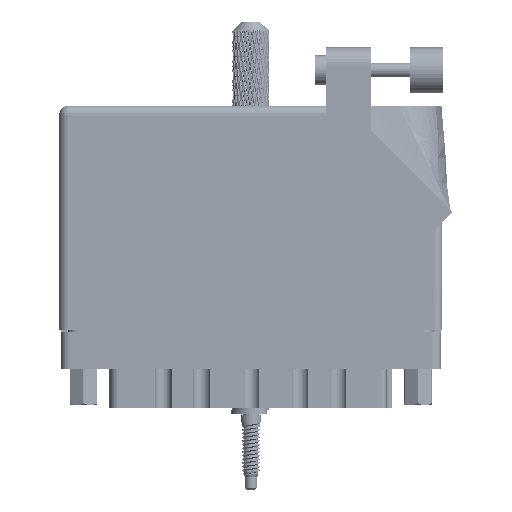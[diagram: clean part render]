
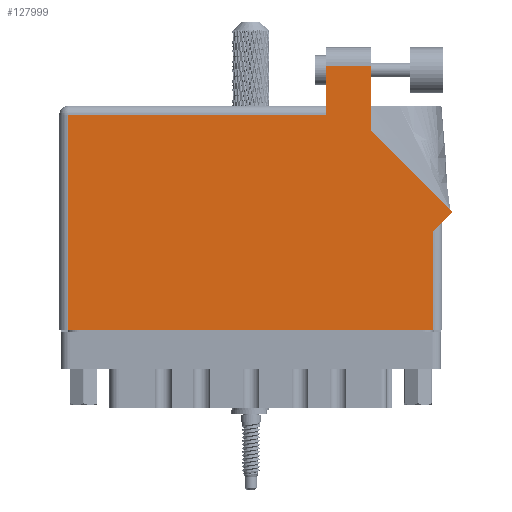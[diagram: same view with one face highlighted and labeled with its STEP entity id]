
A CAD part, front view. The second image highlights one B-rep face of the part: STEP entity #127999.
In plain terms, the highlighted face is planar.
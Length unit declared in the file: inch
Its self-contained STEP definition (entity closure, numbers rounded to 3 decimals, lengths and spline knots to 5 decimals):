
#1914 = DIRECTION ( 'NONE',  ( -1., 0., 0. ) ) ;
#2502 = VECTOR ( 'NONE', #121194, 39.37008 ) ;
#2871 = PLANE ( 'NONE',  #20234 ) ;
#4360 = VERTEX_POINT ( 'NONE', #15477 ) ;
#4693 = ORIENTED_EDGE ( 'NONE', *, *, #49996, .T. ) ;
#5023 = VERTEX_POINT ( 'NONE', #49099 ) ;
#8098 = LINE ( 'NONE', #32141, #100807 ) ;
#8764 = CARTESIAN_POINT ( 'NONE',  ( 1.819, 1.53, 0. ) ) ;
#9034 = VECTOR ( 'NONE', #18438, 39.37008 ) ;
#14349 = FACE_OUTER_BOUND ( 'NONE', #124347, .T. ) ;
#15477 = CARTESIAN_POINT ( 'NONE',  ( 1.819, 1.468, 0. ) ) ;
#15660 = VERTEX_POINT ( 'NONE', #127112 ) ;
#16513 = CARTESIAN_POINT ( 'NONE',  ( 0.062, 0., 0. ) ) ;
#18438 = DIRECTION ( 'NONE',  ( 1., 0., 0. ) ) ;
#19070 = VECTOR ( 'NONE', #127093, 39.37008 ) ;
#20234 = AXIS2_PLACEMENT_3D ( 'NONE', #71954, #51599, #121210 ) ;
#20964 = LINE ( 'NONE', #51165, #2502 ) ;
#21218 = CARTESIAN_POINT ( 'NONE',  ( 2.68271, 0.80771, 0. ) ) ;
#22902 = EDGE_CURVE ( 'NONE', #107381, #66691, #28604, .T. ) ;
#28497 = VERTEX_POINT ( 'NONE', #16513 ) ;
#28604 = LINE ( 'NONE', #21218, #104438 ) ;
#30316 = VERTEX_POINT ( 'NONE', #93687 ) ;
#32141 = CARTESIAN_POINT ( 'NONE',  ( 0.062, 0., 0. ) ) ;
#33255 = LINE ( 'NONE', #126011, #95224 ) ;
#34733 = VECTOR ( 'NONE', #88257, 39.37008 ) ;
#34927 = CARTESIAN_POINT ( 'NONE',  ( 0., 0., 0. ) ) ;
#37935 = EDGE_CURVE ( 'NONE', #4360, #15660, #86525, .T. ) ;
#38525 = EDGE_CURVE ( 'NONE', #30316, #5023, #52386, .T. ) ;
#39911 = DIRECTION ( 'NONE',  ( -1., 0., 0. ) ) ;
#42088 = DIRECTION ( 'NONE',  ( 0., -1., 0. ) ) ;
#42195 = ORIENTED_EDGE ( 'NONE', *, *, #37935, .T. ) ;
#45434 = LINE ( 'NONE', #57933, #19070 ) ;
#49099 = CARTESIAN_POINT ( 'NONE',  ( 1.819, 1.805, 0. ) ) ;
#49996 = EDGE_CURVE ( 'NONE', #111711, #110826, #33255, .T. ) ;
#51165 = CARTESIAN_POINT ( 'NONE',  ( 2.612, 0.737, 0. ) ) ;
#51599 = DIRECTION ( 'NONE',  ( 0., 0., -1. ) ) ;
#52386 = LINE ( 'NONE', #84199, #95732 ) ;
#56889 = ORIENTED_EDGE ( 'NONE', *, *, #96252, .T. ) ;
#57933 = CARTESIAN_POINT ( 'NONE',  ( 2.126, 1.36442, 0. ) ) ;
#65205 = EDGE_CURVE ( 'NONE', #5023, #4360, #87372, .T. ) ;
#66691 = VERTEX_POINT ( 'NONE', #119531 ) ;
#70127 = DIRECTION ( 'NONE',  ( -0.707, 0.707, 0. ) ) ;
#71954 = CARTESIAN_POINT ( 'NONE',  ( 0., 1.53, 0. ) ) ;
#72420 = ORIENTED_EDGE ( 'NONE', *, *, #38525, .T. ) ;
#76337 = CARTESIAN_POINT ( 'NONE',  ( 2.55, 0.675, 0. ) ) ;
#77308 = EDGE_CURVE ( 'NONE', #28497, #111711, #114205, .T. ) ;
#84199 = CARTESIAN_POINT ( 'NONE',  ( 1.819, 1.805, 0. ) ) ;
#84941 = ORIENTED_EDGE ( 'NONE', *, *, #22902, .T. ) ;
#86525 = LINE ( 'NONE', #98291, #120464 ) ;
#87372 = LINE ( 'NONE', #8764, #34733 ) ;
#87773 = CARTESIAN_POINT ( 'NONE',  ( 2.68271, 0.80771, 0. ) ) ;
#88257 = DIRECTION ( 'NONE',  ( 0., -1., 0. ) ) ;
#89093 = EDGE_CURVE ( 'NONE', #66691, #30316, #45434, .T. ) ;
#92206 = ORIENTED_EDGE ( 'NONE', *, *, #89093, .T. ) ;
#93687 = CARTESIAN_POINT ( 'NONE',  ( 2.126, 1.805, 0. ) ) ;
#95224 = VECTOR ( 'NONE', #96217, 39.37008 ) ;
#95732 = VECTOR ( 'NONE', #39911, 39.37008 ) ;
#96217 = DIRECTION ( 'NONE',  ( 0., 1., 0. ) ) ;
#96252 = EDGE_CURVE ( 'NONE', #110826, #107381, #20964, .T. ) ;
#98291 = CARTESIAN_POINT ( 'NONE',  ( 0., 1.468, 0. ) ) ;
#100807 = VECTOR ( 'NONE', #42088, 39.37008 ) ;
#103794 = CARTESIAN_POINT ( 'NONE',  ( 2.55, 0., 0. ) ) ;
#104438 = VECTOR ( 'NONE', #70127, 39.37008 ) ;
#107381 = VERTEX_POINT ( 'NONE', #87773 ) ;
#108740 = EDGE_CURVE ( 'NONE', #15660, #28497, #8098, .T. ) ;
#110826 = VERTEX_POINT ( 'NONE', #76337 ) ;
#111711 = VERTEX_POINT ( 'NONE', #103794 ) ;
#114205 = LINE ( 'NONE', #34927, #9034 ) ;
#114801 = ORIENTED_EDGE ( 'NONE', *, *, #65205, .T. ) ;
#118473 = ORIENTED_EDGE ( 'NONE', *, *, #108740, .T. ) ;
#119531 = CARTESIAN_POINT ( 'NONE',  ( 2.126, 1.36442, 0. ) ) ;
#120464 = VECTOR ( 'NONE', #1914, 39.37008 ) ;
#121194 = DIRECTION ( 'NONE',  ( 0.707, 0.707, 0. ) ) ;
#121210 = DIRECTION ( 'NONE',  ( -1., 0., 0. ) ) ;
#124347 = EDGE_LOOP ( 'NONE', ( #92206, #72420, #114801, #42195, #118473, #127164, #4693, #56889, #84941 ) ) ;
#126011 = CARTESIAN_POINT ( 'NONE',  ( 2.55, 0.737, 0. ) ) ;
#127093 = DIRECTION ( 'NONE',  ( 0., 1., 0. ) ) ;
#127112 = CARTESIAN_POINT ( 'NONE',  ( 0.062, 1.468, 0. ) ) ;
#127164 = ORIENTED_EDGE ( 'NONE', *, *, #77308, .T. ) ;
#127999 = ADVANCED_FACE ( 'NONE', ( #14349 ), #2871, .F. ) ;
